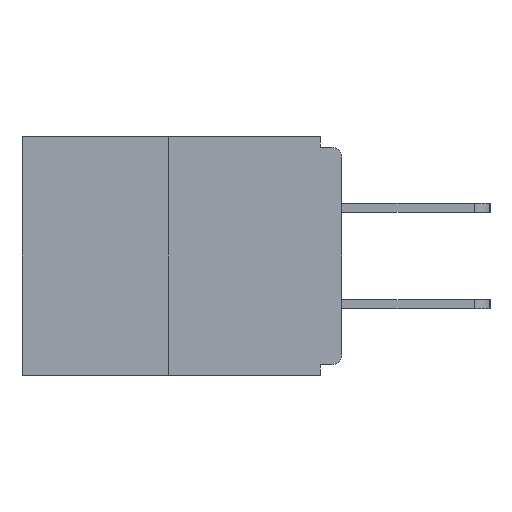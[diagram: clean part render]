
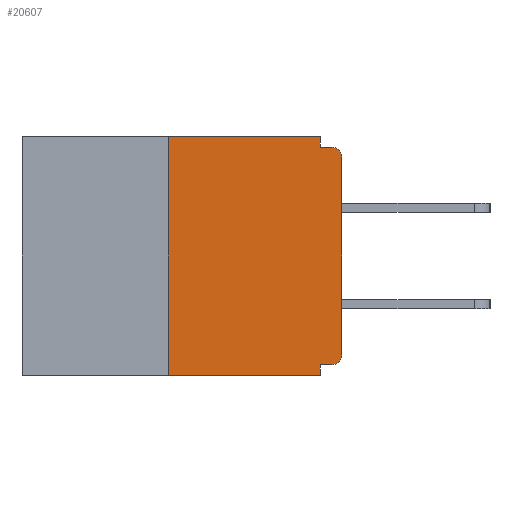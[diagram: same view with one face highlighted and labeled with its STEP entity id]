
A CAD part, left-side view. The second image highlights one B-rep face of the part: STEP entity #20607.
In plain terms, the highlighted planar face has unit normal (-1, 0, 0).
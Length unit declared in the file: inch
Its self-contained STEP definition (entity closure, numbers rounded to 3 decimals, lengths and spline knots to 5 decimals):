
#419 = AXIS2_PLACEMENT_3D ( 'NONE', #1959, #3826, #20264 ) ;
#1720 = LINE ( 'NONE', #11016, #16641 ) ;
#1959 = CARTESIAN_POINT ( 'NONE',  ( 0., 0.46, 0. ) ) ;
#2033 = EDGE_CURVE ( 'NONE', #11212, #25605, #15884, .T. ) ;
#2140 = CARTESIAN_POINT ( 'NONE',  ( 0., 0., -0.03 ) ) ;
#2296 = EDGE_CURVE ( 'NONE', #2874, #6076, #3763, .T. ) ;
#2874 = VERTEX_POINT ( 'NONE', #17155 ) ;
#3463 = CARTESIAN_POINT ( 'NONE',  ( 0., 0.031, -0.328 ) ) ;
#3763 = LINE ( 'NONE', #5409, #8187 ) ;
#3826 = DIRECTION ( 'NONE',  ( 1., 0., 0. ) ) ;
#3859 = ORIENTED_EDGE ( 'NONE', *, *, #2296, .F. ) ;
#4076 = CARTESIAN_POINT ( 'NONE',  ( 0., 0.015, -0.03 ) ) ;
#4143 = ORIENTED_EDGE ( 'NONE', *, *, #8654, .T. ) ;
#4506 = EDGE_CURVE ( 'NONE', #7081, #6049, #9717, .T. ) ;
#4600 = VERTEX_POINT ( 'NONE', #16105 ) ;
#4794 = DIRECTION ( 'NONE',  ( 0., 1., 0. ) ) ;
#5127 = EDGE_CURVE ( 'NONE', #15848, #11134, #17319, .T. ) ;
#5347 = CIRCLE ( 'NONE', #24957, 0.015 ) ;
#5409 = CARTESIAN_POINT ( 'NONE',  ( 0., 0.031, 0. ) ) ;
#5497 = CARTESIAN_POINT ( 'NONE',  ( 0., 0.25, 0. ) ) ;
#6049 = VERTEX_POINT ( 'NONE', #25959 ) ;
#6076 = VERTEX_POINT ( 'NONE', #23511 ) ;
#6460 = DIRECTION ( 'NONE',  ( 0., 0., 1. ) ) ;
#6931 = VECTOR ( 'NONE', #6460, 39.37008 ) ;
#6933 = CARTESIAN_POINT ( 'NONE',  ( 0., 0.015, -0.328 ) ) ;
#6977 = CARTESIAN_POINT ( 'NONE',  ( 0., 0., 0. ) ) ;
#7081 = VERTEX_POINT ( 'NONE', #6933 ) ;
#7481 = EDGE_CURVE ( 'NONE', #7081, #15848, #1720, .T. ) ;
#7549 = CARTESIAN_POINT ( 'NONE',  ( 0., 0.031, -0.343 ) ) ;
#7835 = LINE ( 'NONE', #11758, #23098 ) ;
#7867 = VERTEX_POINT ( 'NONE', #2140 ) ;
#8187 = VECTOR ( 'NONE', #15737, 39.37008 ) ;
#8188 = ORIENTED_EDGE ( 'NONE', *, *, #7481, .F. ) ;
#8510 = ORIENTED_EDGE ( 'NONE', *, *, #12751, .T. ) ;
#8534 = ORIENTED_EDGE ( 'NONE', *, *, #5127, .F. ) ;
#8654 = EDGE_CURVE ( 'NONE', #6049, #7867, #10229, .T. ) ;
#9056 = EDGE_LOOP ( 'NONE', ( #24816, #21944, #8510, #8534, #8188, #19170, #4143, #10311, #17459, #3859 ) ) ;
#9717 = CIRCLE ( 'NONE', #10909, 0.015 ) ;
#10071 = CARTESIAN_POINT ( 'NONE',  ( 0., 0.031, -0.343 ) ) ;
#10229 = LINE ( 'NONE', #6977, #12475 ) ;
#10311 = ORIENTED_EDGE ( 'NONE', *, *, #11428, .T. ) ;
#10909 = AXIS2_PLACEMENT_3D ( 'NONE', #22779, #12410, #24738 ) ;
#11016 = CARTESIAN_POINT ( 'NONE',  ( 0., 0., -0.328 ) ) ;
#11134 = VERTEX_POINT ( 'NONE', #7549 ) ;
#11212 = VERTEX_POINT ( 'NONE', #12483 ) ;
#11428 = EDGE_CURVE ( 'NONE', #7867, #4600, #5347, .T. ) ;
#11758 = CARTESIAN_POINT ( 'NONE',  ( 0., 0.46, 0. ) ) ;
#12410 = DIRECTION ( 'NONE',  ( -1., 0., 0. ) ) ;
#12475 = VECTOR ( 'NONE', #23439, 39.37008 ) ;
#12483 = CARTESIAN_POINT ( 'NONE',  ( 0., 0.25, -0.343 ) ) ;
#12580 = VECTOR ( 'NONE', #20393, 39.37008 ) ;
#12751 = EDGE_CURVE ( 'NONE', #11212, #11134, #14812, .T. ) ;
#13364 = FACE_OUTER_BOUND ( 'NONE', #9056, .T. ) ;
#14812 = LINE ( 'NONE', #17633, #18004 ) ;
#15737 = DIRECTION ( 'NONE',  ( 0., 0., -1. ) ) ;
#15848 = VERTEX_POINT ( 'NONE', #3463 ) ;
#15884 = LINE ( 'NONE', #22747, #6931 ) ;
#16105 = CARTESIAN_POINT ( 'NONE',  ( 0., 0.015, -0.015 ) ) ;
#16641 = VECTOR ( 'NONE', #4794, 39.37008 ) ;
#17155 = CARTESIAN_POINT ( 'NONE',  ( 0., 0.031, 0. ) ) ;
#17319 = LINE ( 'NONE', #10071, #12580 ) ;
#17459 = ORIENTED_EDGE ( 'NONE', *, *, #25207, .F. ) ;
#17633 = CARTESIAN_POINT ( 'NONE',  ( 0., 0.46, -0.343 ) ) ;
#18004 = VECTOR ( 'NONE', #26015, 39.37008 ) ;
#18207 = DIRECTION ( 'NONE',  ( -1., 0., 0. ) ) ;
#19170 = ORIENTED_EDGE ( 'NONE', *, *, #4506, .T. ) ;
#19464 = LINE ( 'NONE', #21965, #25861 ) ;
#19785 = EDGE_CURVE ( 'NONE', #25605, #2874, #7835, .T. ) ;
#20264 = DIRECTION ( 'NONE',  ( 0., 0., -1. ) ) ;
#20393 = DIRECTION ( 'NONE',  ( 0., 0., -1. ) ) ;
#20607 = ADVANCED_FACE ( 'NONE', ( #13364 ), #26161, .F. ) ;
#21944 = ORIENTED_EDGE ( 'NONE', *, *, #2033, .F. ) ;
#21962 = DIRECTION ( 'NONE',  ( 0., -1., 0. ) ) ;
#21965 = CARTESIAN_POINT ( 'NONE',  ( 0., 0., -0.015 ) ) ;
#22747 = CARTESIAN_POINT ( 'NONE',  ( 0., 0.25, 0. ) ) ;
#22779 = CARTESIAN_POINT ( 'NONE',  ( 0., 0.015, -0.313 ) ) ;
#23098 = VECTOR ( 'NONE', #21962, 39.37008 ) ;
#23439 = DIRECTION ( 'NONE',  ( 0., 0., 1. ) ) ;
#23511 = CARTESIAN_POINT ( 'NONE',  ( 0., 0.031, -0.015 ) ) ;
#24148 = DIRECTION ( 'NONE',  ( 0., 0., -1. ) ) ;
#24738 = DIRECTION ( 'NONE',  ( 0., 0., -1. ) ) ;
#24816 = ORIENTED_EDGE ( 'NONE', *, *, #19785, .F. ) ;
#24957 = AXIS2_PLACEMENT_3D ( 'NONE', #4076, #18207, #24148 ) ;
#25207 = EDGE_CURVE ( 'NONE', #6076, #4600, #19464, .T. ) ;
#25605 = VERTEX_POINT ( 'NONE', #5497 ) ;
#25861 = VECTOR ( 'NONE', #26074, 39.37008 ) ;
#25959 = CARTESIAN_POINT ( 'NONE',  ( 0., 0., -0.313 ) ) ;
#26015 = DIRECTION ( 'NONE',  ( 0., -1., 0. ) ) ;
#26074 = DIRECTION ( 'NONE',  ( 0., -1., 0. ) ) ;
#26161 = PLANE ( 'NONE',  #419 ) ;
